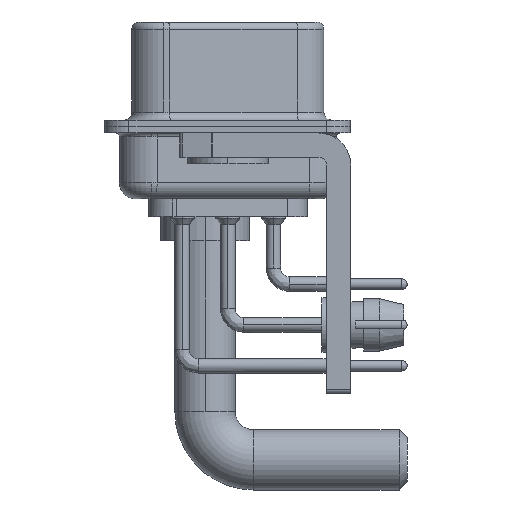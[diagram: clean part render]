
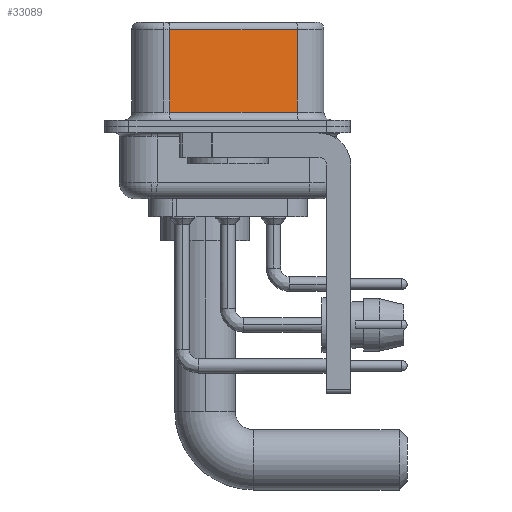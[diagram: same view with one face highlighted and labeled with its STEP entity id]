
A CAD part, left-side view. The second image highlights one B-rep face of the part: STEP entity #33089.
In plain terms, the highlighted planar face has unit normal (-0.985, -0.174, 0).
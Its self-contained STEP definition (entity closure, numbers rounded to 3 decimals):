
#708 = VECTOR ( 'NONE', #39783, 1000. ) ;
#983 = DIRECTION ( 'NONE',  ( -0.174, 0.985, 0. ) ) ;
#1010 = VECTOR ( 'NONE', #11910, 1000. ) ;
#1179 = VECTOR ( 'NONE', #16450, 1000. ) ;
#2032 = EDGE_CURVE ( 'NONE', #11903, #39358, #14520, .T. ) ;
#5226 = ORIENTED_EDGE ( 'NONE', *, *, #28045, .T. ) ;
#5314 = EDGE_LOOP ( 'NONE', ( #25144, #32250, #5226, #5538 ) ) ;
#5538 = ORIENTED_EDGE ( 'NONE', *, *, #6094, .T. ) ;
#6094 = EDGE_CURVE ( 'NONE', #15039, #39358, #16652, .T. ) ;
#8360 = EDGE_CURVE ( 'NONE', #11903, #23232, #18040, .T. ) ;
#10725 = CARTESIAN_POINT ( 'NONE',  ( 3.73, 3.628, 6.52 ) ) ;
#11903 = VERTEX_POINT ( 'NONE', #25467 ) ;
#11910 = DIRECTION ( 'NONE',  ( 0., 0., -1. ) ) ;
#13422 = CARTESIAN_POINT ( 'NONE',  ( 5.132, -4.322, 0.9 ) ) ;
#14520 = LINE ( 'NONE', #33473, #1010 ) ;
#15039 = VERTEX_POINT ( 'NONE', #21555 ) ;
#16450 = DIRECTION ( 'NONE',  ( 0.174, -0.985, 0. ) ) ;
#16652 = LINE ( 'NONE', #13422, #1179 ) ;
#18040 = LINE ( 'NONE', #27711, #708 ) ;
#18651 = CARTESIAN_POINT ( 'NONE',  ( 3.73, 3.628, 6.02 ) ) ;
#18704 = PLANE ( 'NONE',  #30503 ) ;
#21555 = CARTESIAN_POINT ( 'NONE',  ( 3.73, 3.628, 0.9 ) ) ;
#22110 = DIRECTION ( 'NONE',  ( 0.985, 0.174, 0. ) ) ;
#22986 = DIRECTION ( 'NONE',  ( 0., 0., -1. ) ) ;
#23232 = VERTEX_POINT ( 'NONE', #18651 ) ;
#23966 = CARTESIAN_POINT ( 'NONE',  ( 5.132, -4.322, 0.9 ) ) ;
#25144 = ORIENTED_EDGE ( 'NONE', *, *, #2032, .F. ) ;
#25221 = LINE ( 'NONE', #10725, #29628 ) ;
#25467 = CARTESIAN_POINT ( 'NONE',  ( 5.132, -4.322, 6.02 ) ) ;
#27711 = CARTESIAN_POINT ( 'NONE',  ( 5.132, -4.322, 6.02 ) ) ;
#28045 = EDGE_CURVE ( 'NONE', #23232, #15039, #25221, .T. ) ;
#28368 = FACE_OUTER_BOUND ( 'NONE', #5314, .T. ) ;
#29628 = VECTOR ( 'NONE', #22986, 1000. ) ;
#30503 = AXIS2_PLACEMENT_3D ( 'NONE', #37028, #22110, #983 ) ;
#32250 = ORIENTED_EDGE ( 'NONE', *, *, #8360, .T. ) ;
#33089 = ADVANCED_FACE ( 'NONE', ( #28368 ), #18704, .F. ) ;
#33473 = CARTESIAN_POINT ( 'NONE',  ( 5.132, -4.322, 6.52 ) ) ;
#37028 = CARTESIAN_POINT ( 'NONE',  ( 5.132, -4.322, 6.52 ) ) ;
#39358 = VERTEX_POINT ( 'NONE', #23966 ) ;
#39783 = DIRECTION ( 'NONE',  ( -0.174, 0.985, 0. ) ) ;
